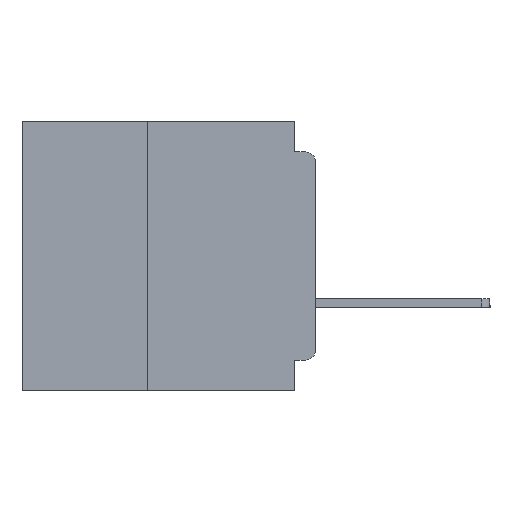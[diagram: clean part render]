
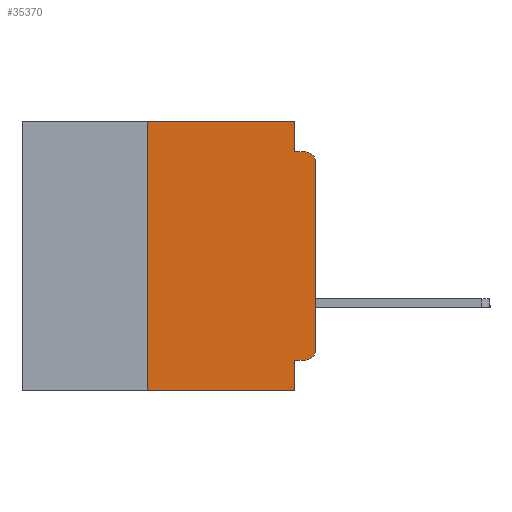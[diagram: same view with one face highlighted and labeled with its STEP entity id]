
A CAD part, left-side view. The second image highlights one B-rep face of the part: STEP entity #35370.
In plain terms, the highlighted planar face has unit normal (-1, 0, 0).
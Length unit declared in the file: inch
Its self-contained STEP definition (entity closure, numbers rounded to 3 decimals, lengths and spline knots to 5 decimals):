
#273 = CARTESIAN_POINT ( 'NONE',  ( 0., 0.031, -0.4 ) ) ;
#1111 = CARTESIAN_POINT ( 'NONE',  ( 0., 0.015, -0.355 ) ) ;
#1183 = CARTESIAN_POINT ( 'NONE',  ( 0., 0., 0. ) ) ;
#2234 = CIRCLE ( 'NONE', #35415, 0.015 ) ;
#2664 = LINE ( 'NONE', #34833, #16642 ) ;
#2846 = FACE_OUTER_BOUND ( 'NONE', #28647, .T. ) ;
#2850 = DIRECTION ( 'NONE',  ( 0., -1., 0. ) ) ;
#3155 = CARTESIAN_POINT ( 'NONE',  ( 0., 0.015, -0.06 ) ) ;
#4353 = LINE ( 'NONE', #22081, #26574 ) ;
#4480 = EDGE_CURVE ( 'NONE', #30364, #5126, #23771, .T. ) ;
#4886 = EDGE_CURVE ( 'NONE', #16883, #29953, #31929, .T. ) ;
#4993 = PLANE ( 'NONE',  #30595 ) ;
#5126 = VERTEX_POINT ( 'NONE', #6354 ) ;
#5380 = DIRECTION ( 'NONE',  ( 0., 1., 0. ) ) ;
#5937 = DIRECTION ( 'NONE',  ( 0., 0., -1. ) ) ;
#5938 = DIRECTION ( 'NONE',  ( 0., -1., 0. ) ) ;
#6354 = CARTESIAN_POINT ( 'NONE',  ( 0., 0., -0.34 ) ) ;
#6684 = VECTOR ( 'NONE', #35246, 39.37008 ) ;
#7767 = DIRECTION ( 'NONE',  ( 1., 0., 0. ) ) ;
#7964 = ORIENTED_EDGE ( 'NONE', *, *, #10750, .F. ) ;
#9664 = EDGE_CURVE ( 'NONE', #31700, #32143, #2234, .T. ) ;
#9791 = VECTOR ( 'NONE', #21496, 39.37008 ) ;
#9898 = EDGE_CURVE ( 'NONE', #13792, #27270, #2664, .T. ) ;
#9913 = LINE ( 'NONE', #1183, #33808 ) ;
#10184 = AXIS2_PLACEMENT_3D ( 'NONE', #27940, #11335, #30709 ) ;
#10750 = EDGE_CURVE ( 'NONE', #30364, #11820, #4353, .T. ) ;
#10937 = CARTESIAN_POINT ( 'NONE',  ( 0., 0.031, -0.355 ) ) ;
#11179 = CARTESIAN_POINT ( 'NONE',  ( 0., 0.437, -0.4 ) ) ;
#11187 = CARTESIAN_POINT ( 'NONE',  ( 0., 0., -0.06 ) ) ;
#11201 = EDGE_CURVE ( 'NONE', #11820, #31755, #18296, .T. ) ;
#11335 = DIRECTION ( 'NONE',  ( -1., 0., 0. ) ) ;
#11820 = VERTEX_POINT ( 'NONE', #10937 ) ;
#11848 = EDGE_CURVE ( 'NONE', #13792, #31755, #35979, .T. ) ;
#12050 = LINE ( 'NONE', #19864, #34157 ) ;
#13792 = VERTEX_POINT ( 'NONE', #18039 ) ;
#15068 = ORIENTED_EDGE ( 'NONE', *, *, #16771, .F. ) ;
#15113 = CARTESIAN_POINT ( 'NONE',  ( 0., 0.25, 0. ) ) ;
#15894 = CARTESIAN_POINT ( 'NONE',  ( 0., 0., -0.045 ) ) ;
#16112 = CARTESIAN_POINT ( 'NONE',  ( 0., 0.437, 0. ) ) ;
#16642 = VECTOR ( 'NONE', #21055, 39.37008 ) ;
#16771 = EDGE_CURVE ( 'NONE', #27270, #16883, #12050, .T. ) ;
#16883 = VERTEX_POINT ( 'NONE', #20227 ) ;
#18039 = CARTESIAN_POINT ( 'NONE',  ( 0., 0.25, -0.4 ) ) ;
#18296 = LINE ( 'NONE', #33273, #32118 ) ;
#18671 = VECTOR ( 'NONE', #2850, 39.37008 ) ;
#18716 = CARTESIAN_POINT ( 'NONE',  ( 0., 0.031, 0. ) ) ;
#18815 = CARTESIAN_POINT ( 'NONE',  ( 0., 0.015, -0.045 ) ) ;
#19864 = CARTESIAN_POINT ( 'NONE',  ( 0., 0.437, 0. ) ) ;
#20227 = CARTESIAN_POINT ( 'NONE',  ( 0., 0.031, 0. ) ) ;
#21055 = DIRECTION ( 'NONE',  ( 0., 0., 1. ) ) ;
#21287 = ORIENTED_EDGE ( 'NONE', *, *, #26774, .T. ) ;
#21496 = DIRECTION ( 'NONE',  ( 0., 0., -1. ) ) ;
#22081 = CARTESIAN_POINT ( 'NONE',  ( 0., 0., -0.355 ) ) ;
#22380 = EDGE_CURVE ( 'NONE', #29953, #32143, #27166, .T. ) ;
#22654 = DIRECTION ( 'NONE',  ( -1., 0., 0. ) ) ;
#23509 = DIRECTION ( 'NONE',  ( 0., 0., 1. ) ) ;
#23771 = CIRCLE ( 'NONE', #10184, 0.015 ) ;
#24123 = ORIENTED_EDGE ( 'NONE', *, *, #9664, .T. ) ;
#26574 = VECTOR ( 'NONE', #5380, 39.37008 ) ;
#26774 = EDGE_CURVE ( 'NONE', #5126, #31700, #9913, .T. ) ;
#27166 = LINE ( 'NONE', #15894, #6684 ) ;
#27258 = ORIENTED_EDGE ( 'NONE', *, *, #9898, .F. ) ;
#27270 = VERTEX_POINT ( 'NONE', #15113 ) ;
#27271 = DIRECTION ( 'NONE',  ( 0., 0., -1. ) ) ;
#27940 = CARTESIAN_POINT ( 'NONE',  ( 0., 0.015, -0.34 ) ) ;
#28647 = EDGE_LOOP ( 'NONE', ( #21287, #24123, #30184, #32765, #15068, #27258, #30831, #29561, #7964, #31902 ) ) ;
#29561 = ORIENTED_EDGE ( 'NONE', *, *, #11201, .F. ) ;
#29953 = VERTEX_POINT ( 'NONE', #35395 ) ;
#30184 = ORIENTED_EDGE ( 'NONE', *, *, #22380, .F. ) ;
#30364 = VERTEX_POINT ( 'NONE', #1111 ) ;
#30595 = AXIS2_PLACEMENT_3D ( 'NONE', #16112, #7767, #27271 ) ;
#30709 = DIRECTION ( 'NONE',  ( 0., 0., -1. ) ) ;
#30831 = ORIENTED_EDGE ( 'NONE', *, *, #11848, .T. ) ;
#31700 = VERTEX_POINT ( 'NONE', #11187 ) ;
#31755 = VERTEX_POINT ( 'NONE', #273 ) ;
#31902 = ORIENTED_EDGE ( 'NONE', *, *, #4480, .T. ) ;
#31929 = LINE ( 'NONE', #18716, #9791 ) ;
#32118 = VECTOR ( 'NONE', #36054, 39.37008 ) ;
#32143 = VERTEX_POINT ( 'NONE', #18815 ) ;
#32765 = ORIENTED_EDGE ( 'NONE', *, *, #4886, .F. ) ;
#33273 = CARTESIAN_POINT ( 'NONE',  ( 0., 0.031, -0.4 ) ) ;
#33808 = VECTOR ( 'NONE', #23509, 39.37008 ) ;
#34157 = VECTOR ( 'NONE', #5938, 39.37008 ) ;
#34833 = CARTESIAN_POINT ( 'NONE',  ( 0., 0.25, -0.4 ) ) ;
#35246 = DIRECTION ( 'NONE',  ( 0., -1., 0. ) ) ;
#35370 = ADVANCED_FACE ( 'NONE', ( #2846 ), #4993, .F. ) ;
#35395 = CARTESIAN_POINT ( 'NONE',  ( 0., 0.031, -0.045 ) ) ;
#35415 = AXIS2_PLACEMENT_3D ( 'NONE', #3155, #22654, #5937 ) ;
#35979 = LINE ( 'NONE', #11179, #18671 ) ;
#36054 = DIRECTION ( 'NONE',  ( 0., 0., -1. ) ) ;
